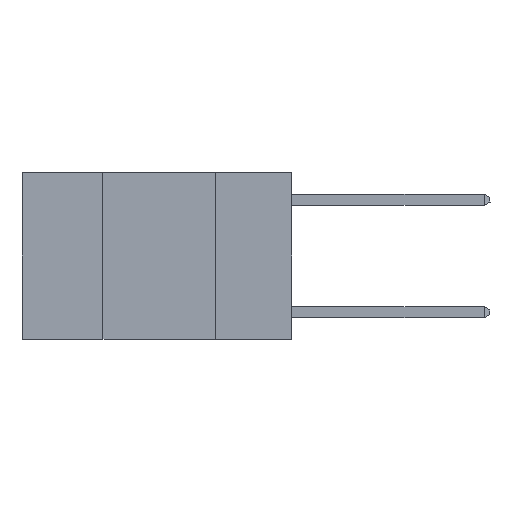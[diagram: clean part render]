
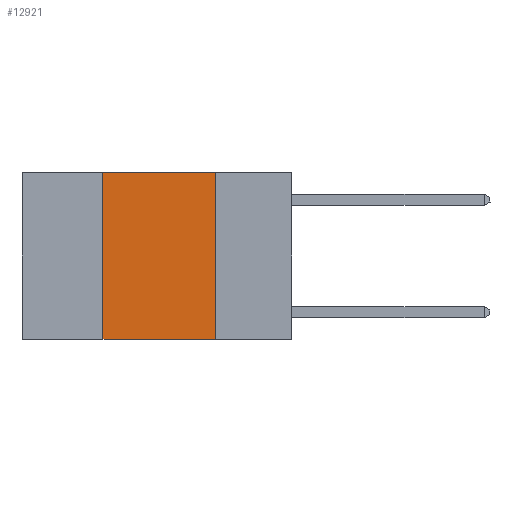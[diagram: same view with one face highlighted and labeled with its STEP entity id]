
A CAD part, left-side view. The second image highlights one B-rep face of the part: STEP entity #12921.
In plain terms, the highlighted planar face has unit normal (-1, 0, 0).
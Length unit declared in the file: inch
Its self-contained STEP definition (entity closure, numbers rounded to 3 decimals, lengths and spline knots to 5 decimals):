
#226 = VERTEX_POINT ( 'NONE', #10953 ) ;
#840 = CARTESIAN_POINT ( 'NONE',  ( 0., 0.6, 0. ) ) ;
#1246 = CARTESIAN_POINT ( 'NONE',  ( 0., 0.42, 0. ) ) ;
#1447 = EDGE_CURVE ( 'NONE', #7247, #226, #17666, .T. ) ;
#3090 = EDGE_CURVE ( 'NONE', #7247, #22059, #3924, .T. ) ;
#3924 = LINE ( 'NONE', #8303, #9635 ) ;
#4730 = EDGE_CURVE ( 'NONE', #19728, #226, #17894, .T. ) ;
#5067 = CARTESIAN_POINT ( 'NONE',  ( 0., 0.6, -0.37 ) ) ;
#6463 = CARTESIAN_POINT ( 'NONE',  ( 0., 0.17, 0. ) ) ;
#7247 = VERTEX_POINT ( 'NONE', #25210 ) ;
#8175 = EDGE_LOOP ( 'NONE', ( #24791, #25251, #25403, #26115 ) ) ;
#8240 = DIRECTION ( 'NONE',  ( 0., 0., -1. ) ) ;
#8303 = CARTESIAN_POINT ( 'NONE',  ( 0., 0.42, 0. ) ) ;
#9635 = VECTOR ( 'NONE', #10843, 39.37008 ) ;
#10843 = DIRECTION ( 'NONE',  ( 0., 0., 1. ) ) ;
#10953 = CARTESIAN_POINT ( 'NONE',  ( 0., 0.17, -0.37 ) ) ;
#12921 = ADVANCED_FACE ( 'NONE', ( #19058 ), #24980, .F. ) ;
#13788 = DIRECTION ( 'NONE',  ( 0., 0., -1. ) ) ;
#13928 = AXIS2_PLACEMENT_3D ( 'NONE', #840, #22683, #8240 ) ;
#14368 = CARTESIAN_POINT ( 'NONE',  ( 0., 0.6, 0. ) ) ;
#16930 = VECTOR ( 'NONE', #24392, 39.37008 ) ;
#16934 = DIRECTION ( 'NONE',  ( 0., -1., 0. ) ) ;
#17666 = LINE ( 'NONE', #5067, #16930 ) ;
#17894 = LINE ( 'NONE', #6463, #22743 ) ;
#19058 = FACE_OUTER_BOUND ( 'NONE', #8175, .T. ) ;
#19728 = VERTEX_POINT ( 'NONE', #30516 ) ;
#22059 = VERTEX_POINT ( 'NONE', #1246 ) ;
#22683 = DIRECTION ( 'NONE',  ( 1., 0., 0. ) ) ;
#22743 = VECTOR ( 'NONE', #13788, 39.37008 ) ;
#24392 = DIRECTION ( 'NONE',  ( 0., -1., 0. ) ) ;
#24791 = ORIENTED_EDGE ( 'NONE', *, *, #4730, .F. ) ;
#24980 = PLANE ( 'NONE',  #13928 ) ;
#25210 = CARTESIAN_POINT ( 'NONE',  ( 0., 0.42, -0.37 ) ) ;
#25251 = ORIENTED_EDGE ( 'NONE', *, *, #27241, .F. ) ;
#25403 = ORIENTED_EDGE ( 'NONE', *, *, #3090, .F. ) ;
#26115 = ORIENTED_EDGE ( 'NONE', *, *, #1447, .T. ) ;
#27241 = EDGE_CURVE ( 'NONE', #22059, #19728, #28499, .T. ) ;
#27779 = VECTOR ( 'NONE', #16934, 39.37008 ) ;
#28499 = LINE ( 'NONE', #14368, #27779 ) ;
#30516 = CARTESIAN_POINT ( 'NONE',  ( 0., 0.17, 0. ) ) ;
